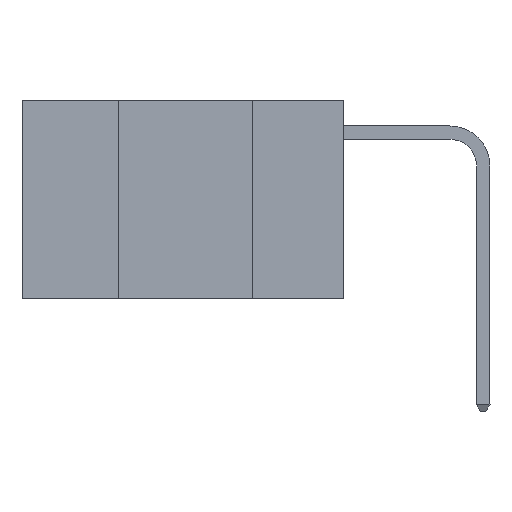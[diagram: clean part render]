
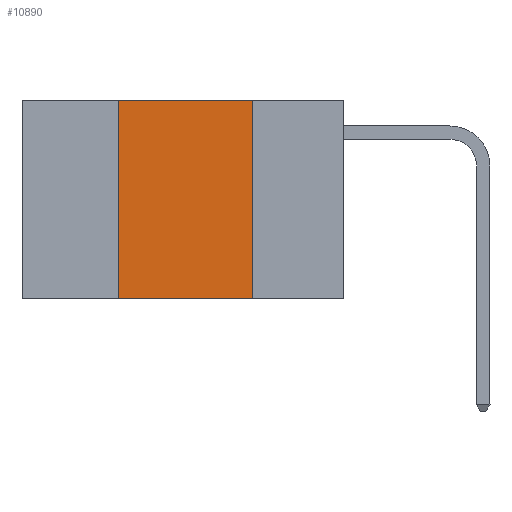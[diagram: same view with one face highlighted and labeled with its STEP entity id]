
A CAD part, left-side view. The second image highlights one B-rep face of the part: STEP entity #10890.
In plain terms, the highlighted planar face has unit normal (-1, 0, 0).
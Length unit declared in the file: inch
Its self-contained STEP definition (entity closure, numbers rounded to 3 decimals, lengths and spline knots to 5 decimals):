
#809 = LINE ( 'NONE', #3326, #921 ) ;
#843 = AXIS2_PLACEMENT_3D ( 'NONE', #1894, #3118, #10306 ) ;
#921 = VECTOR ( 'NONE', #3321, 39.37008 ) ;
#1127 = CARTESIAN_POINT ( 'NONE',  ( 0., 0.6, 0. ) ) ;
#1156 = DIRECTION ( 'NONE',  ( 0., -1., 0. ) ) ;
#1274 = EDGE_LOOP ( 'NONE', ( #7693, #7848, #7897, #7907 ) ) ;
#1894 = CARTESIAN_POINT ( 'NONE',  ( 0., 0.6, 0. ) ) ;
#3118 = DIRECTION ( 'NONE',  ( 1., 0., 0. ) ) ;
#3168 = VERTEX_POINT ( 'NONE', #6582 ) ;
#3297 = EDGE_CURVE ( 'NONE', #3310, #10190, #11380, .T. ) ;
#3310 = VERTEX_POINT ( 'NONE', #5461 ) ;
#3321 = DIRECTION ( 'NONE',  ( 0., 0., 1. ) ) ;
#3326 = CARTESIAN_POINT ( 'NONE',  ( 0., 0.42, 0. ) ) ;
#3905 = CARTESIAN_POINT ( 'NONE',  ( 0., 0.42, 0. ) ) ;
#4710 = DIRECTION ( 'NONE',  ( 0., -1., 0. ) ) ;
#5312 = VERTEX_POINT ( 'NONE', #3905 ) ;
#5461 = CARTESIAN_POINT ( 'NONE',  ( 0., 0.17, 0. ) ) ;
#5496 = VECTOR ( 'NONE', #4710, 39.37008 ) ;
#5530 = CARTESIAN_POINT ( 'NONE',  ( 0., 0.17, 0. ) ) ;
#5533 = DIRECTION ( 'NONE',  ( 0., 0., -1. ) ) ;
#5580 = LINE ( 'NONE', #5843, #5496 ) ;
#5843 = CARTESIAN_POINT ( 'NONE',  ( 0., 0.6, -0.37 ) ) ;
#6582 = CARTESIAN_POINT ( 'NONE',  ( 0., 0.42, -0.37 ) ) ;
#7065 = CARTESIAN_POINT ( 'NONE',  ( 0., 0.17, -0.37 ) ) ;
#7693 = ORIENTED_EDGE ( 'NONE', *, *, #3297, .F. ) ;
#7848 = ORIENTED_EDGE ( 'NONE', *, *, #8210, .F. ) ;
#7897 = ORIENTED_EDGE ( 'NONE', *, *, #7900, .F. ) ;
#7900 = EDGE_CURVE ( 'NONE', #3168, #5312, #809, .T. ) ;
#7907 = ORIENTED_EDGE ( 'NONE', *, *, #9003, .T. ) ;
#8210 = EDGE_CURVE ( 'NONE', #5312, #3310, #8826, .T. ) ;
#8437 = PLANE ( 'NONE',  #843 ) ;
#8539 = VECTOR ( 'NONE', #1156, 39.37008 ) ;
#8826 = LINE ( 'NONE', #1127, #8539 ) ;
#9003 = EDGE_CURVE ( 'NONE', #3168, #10190, #5580, .T. ) ;
#10190 = VERTEX_POINT ( 'NONE', #7065 ) ;
#10306 = DIRECTION ( 'NONE',  ( 0., 0., -1. ) ) ;
#10890 = ADVANCED_FACE ( 'NONE', ( #12838 ), #8437, .F. ) ;
#11380 = LINE ( 'NONE', #5530, #11456 ) ;
#11456 = VECTOR ( 'NONE', #5533, 39.37008 ) ;
#12838 = FACE_OUTER_BOUND ( 'NONE', #1274, .T. ) ;
